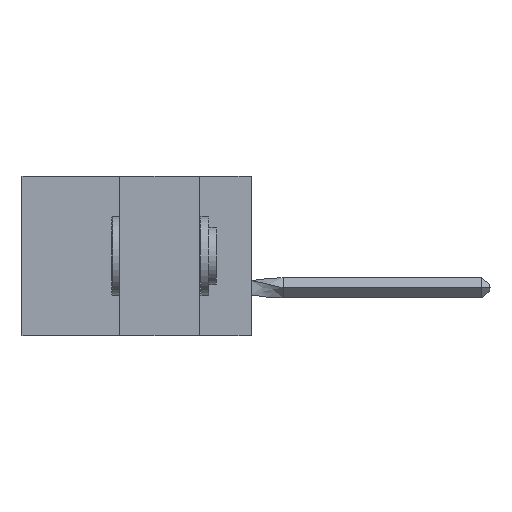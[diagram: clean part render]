
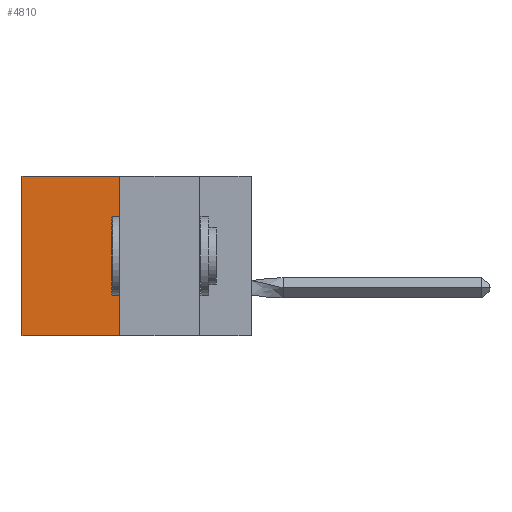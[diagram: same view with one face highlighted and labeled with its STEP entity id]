
A CAD part, left-side view. The second image highlights one B-rep face of the part: STEP entity #4810.
In plain terms, the highlighted planar face has unit normal (-1, 0, 0).
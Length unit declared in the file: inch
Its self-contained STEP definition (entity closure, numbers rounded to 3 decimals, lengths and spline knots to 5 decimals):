
#258 = CARTESIAN_POINT ( 'NONE',  ( 0.305, 0.413, 0. ) ) ;
#1642 = VECTOR ( 'NONE', #6435, 39.37008 ) ;
#2215 = FACE_OUTER_BOUND ( 'NONE', #22110, .T. ) ;
#3090 = CARTESIAN_POINT ( 'NONE',  ( 0.305, 0.72, -0.5 ) ) ;
#3142 = EDGE_CURVE ( 'NONE', #38987, #6170, #38706, .T. ) ;
#4560 = LINE ( 'NONE', #3090, #32376 ) ;
#4810 = ADVANCED_FACE ( 'NONE', ( #2215 ), #27249, .F. ) ;
#6037 = CARTESIAN_POINT ( 'NONE',  ( 0.305, 0.413, 0. ) ) ;
#6170 = VERTEX_POINT ( 'NONE', #15087 ) ;
#6435 = DIRECTION ( 'NONE',  ( 0., 1., 0. ) ) ;
#10074 = ORIENTED_EDGE ( 'NONE', *, *, #3142, .T. ) ;
#15087 = CARTESIAN_POINT ( 'NONE',  ( 0.305, 0.72, 0. ) ) ;
#15340 = CARTESIAN_POINT ( 'NONE',  ( 0.305, 0.413, -0.5 ) ) ;
#15637 = VERTEX_POINT ( 'NONE', #27472 ) ;
#15704 = DIRECTION ( 'NONE',  ( 0., 0., -1. ) ) ;
#18035 = CARTESIAN_POINT ( 'NONE',  ( 0.305, 0.72, -0.5 ) ) ;
#18747 = LINE ( 'NONE', #35741, #28837 ) ;
#19648 = EDGE_CURVE ( 'NONE', #6170, #23727, #4560, .T. ) ;
#19990 = DIRECTION ( 'NONE',  ( 0., 0., -1. ) ) ;
#22006 = EDGE_CURVE ( 'NONE', #38987, #15637, #18747, .T. ) ;
#22110 = EDGE_LOOP ( 'NONE', ( #26751, #23315, #29389, #10074 ) ) ;
#23315 = ORIENTED_EDGE ( 'NONE', *, *, #25921, .F. ) ;
#23351 = LINE ( 'NONE', #35341, #34471 ) ;
#23682 = AXIS2_PLACEMENT_3D ( 'NONE', #15340, #33650, #39867 ) ;
#23727 = VERTEX_POINT ( 'NONE', #18035 ) ;
#25921 = EDGE_CURVE ( 'NONE', #15637, #23727, #23351, .T. ) ;
#26751 = ORIENTED_EDGE ( 'NONE', *, *, #19648, .T. ) ;
#27249 = PLANE ( 'NONE',  #23682 ) ;
#27472 = CARTESIAN_POINT ( 'NONE',  ( 0.305, 0.413, -0.5 ) ) ;
#28837 = VECTOR ( 'NONE', #19990, 39.37008 ) ;
#29389 = ORIENTED_EDGE ( 'NONE', *, *, #22006, .F. ) ;
#32376 = VECTOR ( 'NONE', #15704, 39.37008 ) ;
#33650 = DIRECTION ( 'NONE',  ( 1., 0., 0. ) ) ;
#34471 = VECTOR ( 'NONE', #36284, 39.37008 ) ;
#35341 = CARTESIAN_POINT ( 'NONE',  ( 0.305, 0.413, -0.5 ) ) ;
#35741 = CARTESIAN_POINT ( 'NONE',  ( 0.305, 0.413, -0.5 ) ) ;
#36284 = DIRECTION ( 'NONE',  ( 0., 1., 0. ) ) ;
#38706 = LINE ( 'NONE', #258, #1642 ) ;
#38987 = VERTEX_POINT ( 'NONE', #6037 ) ;
#39867 = DIRECTION ( 'NONE',  ( 0., 0., -1. ) ) ;
